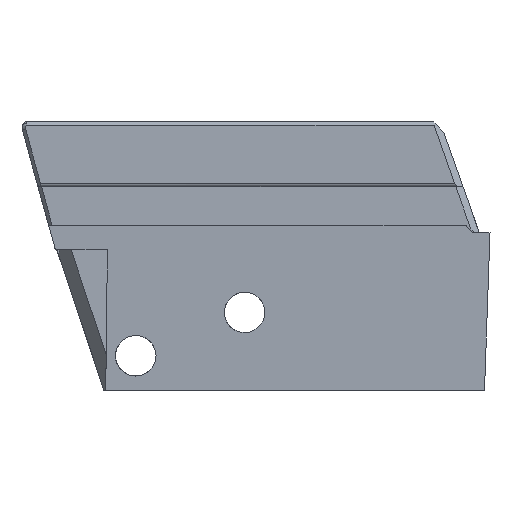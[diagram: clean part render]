
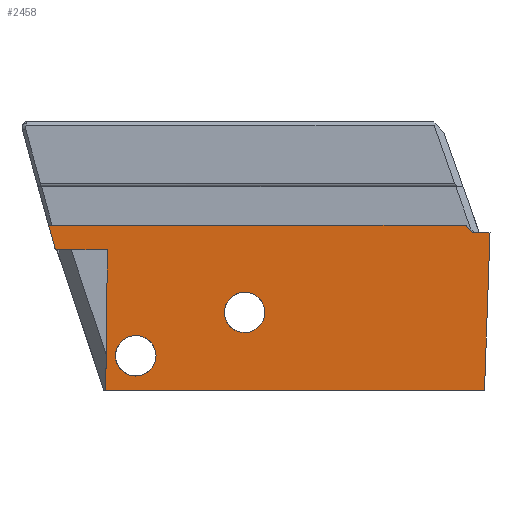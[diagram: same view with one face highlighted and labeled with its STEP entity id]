
A CAD part, front view. The second image highlights one B-rep face of the part: STEP entity #2458.
In plain terms, the highlighted planar face has unit normal (0, -0.999, -0.035).
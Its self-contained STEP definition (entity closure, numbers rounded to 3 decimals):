
#26=FACE_BOUND('',#373,.T.);
#27=FACE_BOUND('',#374,.T.);
#67=(
BOUNDED_CURVE()
B_SPLINE_CURVE(2,(#3966,#3967,#3968),.UNSPECIFIED.,.F.,.F.)
B_SPLINE_CURVE_WITH_KNOTS((3,3),(-1.868,-1.786),
 .UNSPECIFIED.)
CURVE()
GEOMETRIC_REPRESENTATION_ITEM()
RATIONAL_B_SPLINE_CURVE((1.,1.,1.))
REPRESENTATION_ITEM('')
);
#132=PLANE('',#2623);
#242=FACE_OUTER_BOUND('',#372,.T.);
#372=EDGE_LOOP('',(#1951,#1952,#1953,#1954,#1955,#1956,#1957,#1958));
#373=EDGE_LOOP('',(#1959));
#374=EDGE_LOOP('',(#1960));
#503=LINE('',#3462,#788);
#559=LINE('',#3843,#844);
#606=LINE('',#3960,#891);
#607=LINE('',#3962,#892);
#608=LINE('',#3964,#893);
#609=LINE('',#3969,#894);
#610=LINE('',#3970,#895);
#788=VECTOR('',#2823,1000.);
#844=VECTOR('',#2927,1000.);
#891=VECTOR('',#3018,1000.);
#892=VECTOR('',#3019,1000.);
#893=VECTOR('',#3020,1000.);
#894=VECTOR('',#3021,1000.);
#895=VECTOR('',#3022,1000.);
#1035=ELLIPSE('',#2610,1.501,1.5);
#1036=ELLIPSE('',#2612,1.501,1.5);
#1095=VERTEX_POINT('',#3459);
#1096=VERTEX_POINT('',#3461);
#1159=VERTEX_POINT('',#3840);
#1160=VERTEX_POINT('',#3842);
#1170=VERTEX_POINT('',#3878);
#1171=VERTEX_POINT('',#3882);
#1198=VERTEX_POINT('',#3959);
#1199=VERTEX_POINT('',#3961);
#1200=VERTEX_POINT('',#3963);
#1201=VERTEX_POINT('',#3965);
#1354=EDGE_CURVE('',#1095,#1096,#503,.T.);
#1432=EDGE_CURVE('',#1159,#1160,#559,.T.);
#1452=EDGE_CURVE('',#1170,#1170,#1035,.T.);
#1454=EDGE_CURVE('',#1171,#1171,#1036,.T.);
#1488=EDGE_CURVE('',#1160,#1198,#606,.T.);
#1489=EDGE_CURVE('',#1159,#1199,#607,.T.);
#1490=EDGE_CURVE('',#1200,#1199,#608,.T.);
#1491=EDGE_CURVE('',#1201,#1200,#67,.T.);
#1492=EDGE_CURVE('',#1096,#1201,#609,.T.);
#1493=EDGE_CURVE('',#1198,#1095,#610,.T.);
#1951=ORIENTED_EDGE('',*,*,#1488,.F.);
#1952=ORIENTED_EDGE('',*,*,#1432,.F.);
#1953=ORIENTED_EDGE('',*,*,#1489,.T.);
#1954=ORIENTED_EDGE('',*,*,#1490,.F.);
#1955=ORIENTED_EDGE('',*,*,#1491,.F.);
#1956=ORIENTED_EDGE('',*,*,#1492,.F.);
#1957=ORIENTED_EDGE('',*,*,#1354,.F.);
#1958=ORIENTED_EDGE('',*,*,#1493,.F.);
#1959=ORIENTED_EDGE('',*,*,#1452,.T.);
#1960=ORIENTED_EDGE('',*,*,#1454,.T.);
#2458=ADVANCED_FACE('',(#242,#26,#27),#132,.F.);
#2610=AXIS2_PLACEMENT_3D('',#3879,#2961,#2962);
#2612=AXIS2_PLACEMENT_3D('',#3883,#2966,#2967);
#2623=AXIS2_PLACEMENT_3D('',#3958,#3016,#3017);
#2823=DIRECTION('',(-0.266,-0.034,0.963));
#2927=DIRECTION('',(-1.,0.,0.));
#2961=DIRECTION('center_axis',(0.,0.999,0.035));
#2962=DIRECTION('ref_axis',(0.,-0.035,0.999));
#2966=DIRECTION('center_axis',(0.,0.999,0.035));
#2967=DIRECTION('ref_axis',(0.,-0.035,0.999));
#3016=DIRECTION('center_axis',(0.,0.999,0.035));
#3017=DIRECTION('ref_axis',(1.,0.,0.));
#3018=DIRECTION('',(0.012,-0.035,0.999));
#3019=DIRECTION('',(0.035,-0.035,0.999));
#3020=DIRECTION('',(1.,0.,0.));
#3021=DIRECTION('',(1.,0.,0.));
#3022=DIRECTION('',(-1.,0.,0.));
#3459=CARTESIAN_POINT('',(-14.964,59.539,-1.939));
#3461=CARTESIAN_POINT('',(-15.472,59.474,-0.1));
#3462=CARTESIAN_POINT('',(-14.307,59.622,-4.319));
#3840=CARTESIAN_POINT('',(16.799,59.901,-12.321));
#3842=CARTESIAN_POINT('',(-11.243,59.901,-12.321));
#3843=CARTESIAN_POINT('',(32.,59.901,-12.321));
#3878=CARTESIAN_POINT('',(-7.521,59.812,-9.772));
#3879=CARTESIAN_POINT('Origin',(-9.021,59.812,-9.772));
#3882=CARTESIAN_POINT('',(0.542,59.7,-6.559));
#3883=CARTESIAN_POINT('Origin',(-0.958,59.7,-6.559));
#3958=CARTESIAN_POINT('Origin',(-15.472,59.366,2.998));
#3959=CARTESIAN_POINT('',(-11.122,59.539,-1.939));
#3960=CARTESIAN_POINT('',(-11.073,59.394,2.193));
#3961=CARTESIAN_POINT('',(17.207,59.494,-0.654));
#3962=CARTESIAN_POINT('',(17.294,59.406,1.851));
#3963=CARTESIAN_POINT('',(15.921,59.494,-0.654));
#3964=CARTESIAN_POINT('',(-87.009,59.494,-0.654));
#3965=CARTESIAN_POINT('',(15.363,59.474,-0.1));
#3966=CARTESIAN_POINT('Ctrl Pts',(15.363,59.474,-0.1));
#3967=CARTESIAN_POINT('Ctrl Pts',(15.641,59.484,-0.376));
#3968=CARTESIAN_POINT('Ctrl Pts',(15.921,59.494,-0.654));
#3969=CARTESIAN_POINT('',(-70.172,59.474,-0.1));
#3970=CARTESIAN_POINT('',(-15.472,59.539,-1.939));
